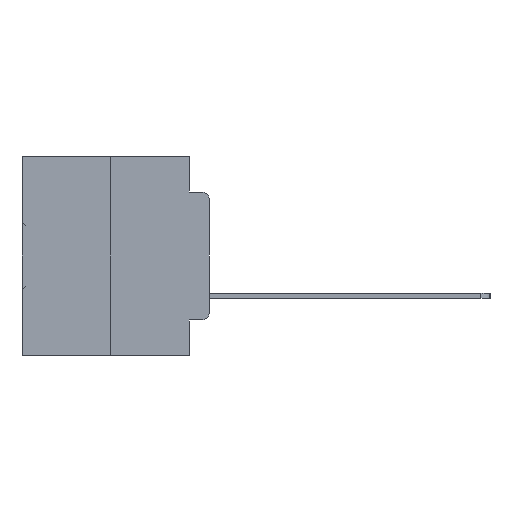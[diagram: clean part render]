
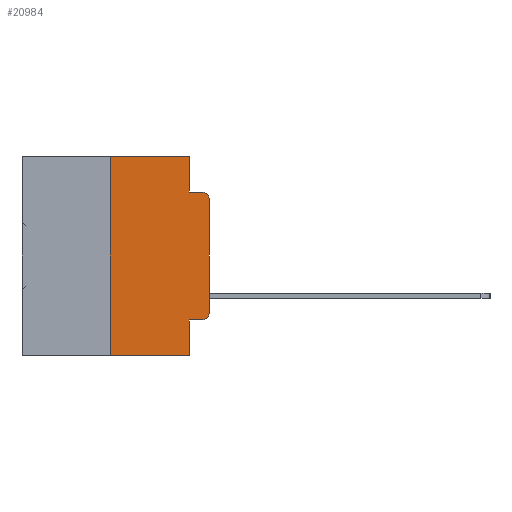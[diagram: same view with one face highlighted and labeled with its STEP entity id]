
A CAD part, left-side view. The second image highlights one B-rep face of the part: STEP entity #20984.
In plain terms, the highlighted planar face has unit normal (-1, 0, 0).
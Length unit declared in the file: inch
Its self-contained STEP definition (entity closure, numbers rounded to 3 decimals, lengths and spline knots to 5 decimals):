
#530 = DIRECTION ( 'NONE',  ( -1., 0., 0. ) ) ;
#1120 = ORIENTED_EDGE ( 'NONE', *, *, #31228, .T. ) ;
#1331 = CARTESIAN_POINT ( 'NONE',  ( 0., 0.051, 0. ) ) ;
#1355 = VERTEX_POINT ( 'NONE', #14260 ) ;
#2441 = VERTEX_POINT ( 'NONE', #28019 ) ;
#2850 = LINE ( 'NONE', #23960, #17153 ) ;
#3449 = ORIENTED_EDGE ( 'NONE', *, *, #31525, .T. ) ;
#3732 = CARTESIAN_POINT ( 'NONE',  ( 0., 0., 0. ) ) ;
#3850 = ORIENTED_EDGE ( 'NONE', *, *, #13308, .F. ) ;
#4632 = ORIENTED_EDGE ( 'NONE', *, *, #16898, .T. ) ;
#4643 = VECTOR ( 'NONE', #33073, 39.37008 ) ;
#4991 = LINE ( 'NONE', #5535, #11369 ) ;
#5191 = CARTESIAN_POINT ( 'NONE',  ( 0., 0.25, 0. ) ) ;
#5535 = CARTESIAN_POINT ( 'NONE',  ( 0., 0.25, 0. ) ) ;
#5605 = VERTEX_POINT ( 'NONE', #9875 ) ;
#5870 = LINE ( 'NONE', #1331, #13026 ) ;
#6035 = VECTOR ( 'NONE', #31496, 39.37008 ) ;
#6153 = EDGE_CURVE ( 'NONE', #1355, #30666, #20971, .T. ) ;
#7461 = VERTEX_POINT ( 'NONE', #25286 ) ;
#7687 = AXIS2_PLACEMENT_3D ( 'NONE', #31202, #15569, #33753 ) ;
#8006 = EDGE_CURVE ( 'NONE', #15032, #1355, #5870, .T. ) ;
#8021 = CARTESIAN_POINT ( 'NONE',  ( 0., 0.02, -0.0885 ) ) ;
#8585 = VECTOR ( 'NONE', #22368, 39.37008 ) ;
#9875 = CARTESIAN_POINT ( 'NONE',  ( 0., 0.051, -0.5 ) ) ;
#11369 = VECTOR ( 'NONE', #13657, 39.37008 ) ;
#11521 = DIRECTION ( 'NONE',  ( -1., 0., 0. ) ) ;
#11528 = LINE ( 'NONE', #13221, #6035 ) ;
#12339 = ORIENTED_EDGE ( 'NONE', *, *, #8006, .F. ) ;
#13026 = VECTOR ( 'NONE', #17466, 39.37008 ) ;
#13221 = CARTESIAN_POINT ( 'NONE',  ( 0., 0.473, -0.5 ) ) ;
#13269 = CARTESIAN_POINT ( 'NONE',  ( 0., 0.051, 0. ) ) ;
#13308 = EDGE_CURVE ( 'NONE', #2441, #16158, #4991, .T. ) ;
#13616 = ORIENTED_EDGE ( 'NONE', *, *, #17253, .T. ) ;
#13657 = DIRECTION ( 'NONE',  ( 0., 0., 1. ) ) ;
#13728 = CARTESIAN_POINT ( 'NONE',  ( 0., 0.051, -0.4115 ) ) ;
#13941 = ORIENTED_EDGE ( 'NONE', *, *, #15835, .T. ) ;
#14260 = CARTESIAN_POINT ( 'NONE',  ( 0., 0.051, -0.0885 ) ) ;
#14426 = EDGE_LOOP ( 'NONE', ( #3449, #4632, #25704, #12339, #22629, #3850, #1120, #26980, #13616, #13941 ) ) ;
#14834 = VECTOR ( 'NONE', #25970, 39.37008 ) ;
#15032 = VERTEX_POINT ( 'NONE', #13269 ) ;
#15141 = VERTEX_POINT ( 'NONE', #13728 ) ;
#15569 = DIRECTION ( 'NONE',  ( 1., 0., 0. ) ) ;
#15835 = EDGE_CURVE ( 'NONE', #24670, #7461, #23594, .T. ) ;
#16158 = VERTEX_POINT ( 'NONE', #5191 ) ;
#16682 = CARTESIAN_POINT ( 'NONE',  ( 0., 0.02, -0.3915 ) ) ;
#16898 = EDGE_CURVE ( 'NONE', #31087, #30666, #26339, .T. ) ;
#17153 = VECTOR ( 'NONE', #34193, 39.37008 ) ;
#17253 = EDGE_CURVE ( 'NONE', #15141, #24670, #28779, .T. ) ;
#17346 = DIRECTION ( 'NONE',  ( 0., -1., 0. ) ) ;
#17466 = DIRECTION ( 'NONE',  ( 0., 0., -1. ) ) ;
#19085 = AXIS2_PLACEMENT_3D ( 'NONE', #16682, #530, #19311 ) ;
#19311 = DIRECTION ( 'NONE',  ( 0., 0., -1. ) ) ;
#20971 = LINE ( 'NONE', #27734, #27913 ) ;
#20984 = ADVANCED_FACE ( 'NONE', ( #32487 ), #28631, .F. ) ;
#22368 = DIRECTION ( 'NONE',  ( 0., 0., 1. ) ) ;
#22498 = EDGE_CURVE ( 'NONE', #15141, #5605, #2850, .T. ) ;
#22629 = ORIENTED_EDGE ( 'NONE', *, *, #32237, .F. ) ;
#23594 = CIRCLE ( 'NONE', #19085, 0.02 ) ;
#23960 = CARTESIAN_POINT ( 'NONE',  ( 0., 0.051, 0. ) ) ;
#24670 = VERTEX_POINT ( 'NONE', #25733 ) ;
#25286 = CARTESIAN_POINT ( 'NONE',  ( 0., 0., -0.3915 ) ) ;
#25704 = ORIENTED_EDGE ( 'NONE', *, *, #6153, .F. ) ;
#25730 = CARTESIAN_POINT ( 'NONE',  ( 0., 0., -0.1085 ) ) ;
#25733 = CARTESIAN_POINT ( 'NONE',  ( 0., 0.02, -0.4115 ) ) ;
#25970 = DIRECTION ( 'NONE',  ( 0., -1., 0. ) ) ;
#26339 = CIRCLE ( 'NONE', #32807, 0.02 ) ;
#26980 = ORIENTED_EDGE ( 'NONE', *, *, #22498, .F. ) ;
#27242 = CARTESIAN_POINT ( 'NONE',  ( 0., 0.02, -0.1085 ) ) ;
#27734 = CARTESIAN_POINT ( 'NONE',  ( 0., 0.051, -0.0885 ) ) ;
#27913 = VECTOR ( 'NONE', #17346, 39.37008 ) ;
#28019 = CARTESIAN_POINT ( 'NONE',  ( 0., 0.25, -0.5 ) ) ;
#28631 = PLANE ( 'NONE',  #7687 ) ;
#28748 = LINE ( 'NONE', #3732, #8585 ) ;
#28779 = LINE ( 'NONE', #33621, #14834 ) ;
#29832 = DIRECTION ( 'NONE',  ( 0., 0., -1. ) ) ;
#30517 = CARTESIAN_POINT ( 'NONE',  ( 0., 0.473, 0. ) ) ;
#30666 = VERTEX_POINT ( 'NONE', #8021 ) ;
#31087 = VERTEX_POINT ( 'NONE', #25730 ) ;
#31202 = CARTESIAN_POINT ( 'NONE',  ( 0., 0.473, 0. ) ) ;
#31228 = EDGE_CURVE ( 'NONE', #2441, #5605, #11528, .T. ) ;
#31496 = DIRECTION ( 'NONE',  ( 0., -1., 0. ) ) ;
#31525 = EDGE_CURVE ( 'NONE', #7461, #31087, #28748, .T. ) ;
#32237 = EDGE_CURVE ( 'NONE', #16158, #15032, #32671, .T. ) ;
#32487 = FACE_OUTER_BOUND ( 'NONE', #14426, .T. ) ;
#32671 = LINE ( 'NONE', #30517, #4643 ) ;
#32807 = AXIS2_PLACEMENT_3D ( 'NONE', #27242, #11521, #29832 ) ;
#33073 = DIRECTION ( 'NONE',  ( 0., -1., 0. ) ) ;
#33621 = CARTESIAN_POINT ( 'NONE',  ( 0., 0.051, -0.4115 ) ) ;
#33753 = DIRECTION ( 'NONE',  ( 0., 0., -1. ) ) ;
#34193 = DIRECTION ( 'NONE',  ( 0., 0., -1. ) ) ;
